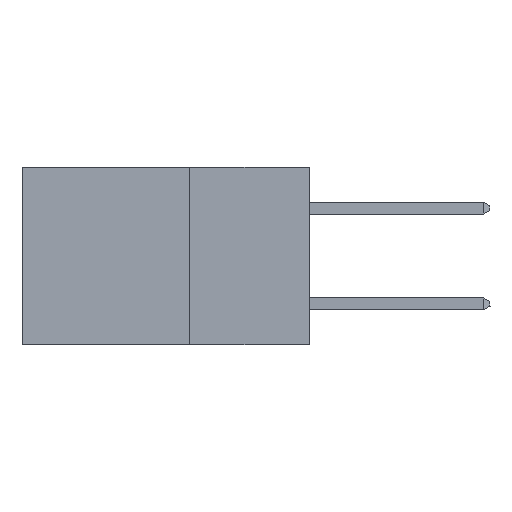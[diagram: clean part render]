
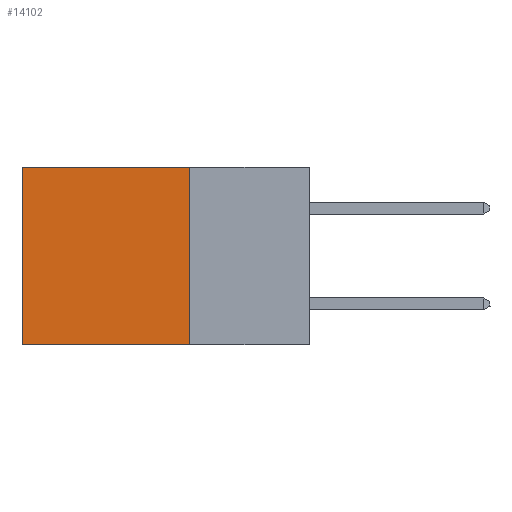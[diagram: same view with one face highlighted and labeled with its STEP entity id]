
A CAD part, left-side view. The second image highlights one B-rep face of the part: STEP entity #14102.
In plain terms, the highlighted planar face has unit normal (-1, 0, 0).
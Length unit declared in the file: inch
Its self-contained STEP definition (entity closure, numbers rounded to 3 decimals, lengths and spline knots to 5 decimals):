
#284 = VERTEX_POINT ( 'NONE', #14737 ) ;
#2550 = LINE ( 'NONE', #11551, #12801 ) ;
#3171 = ORIENTED_EDGE ( 'NONE', *, *, #9326, .T. ) ;
#3224 = ORIENTED_EDGE ( 'NONE', *, *, #5457, .F. ) ;
#3349 = ORIENTED_EDGE ( 'NONE', *, *, #16497, .F. ) ;
#3439 = CARTESIAN_POINT ( 'NONE',  ( 0.2875, 0.25, -0.37 ) ) ;
#3524 = CARTESIAN_POINT ( 'NONE',  ( 0.2875, 0.25, -0.37 ) ) ;
#4441 = AXIS2_PLACEMENT_3D ( 'NONE', #5924, #4626, #13825 ) ;
#4534 = EDGE_CURVE ( 'NONE', #12306, #284, #9632, .T. ) ;
#4618 = DIRECTION ( 'NONE',  ( 0., 1., 0. ) ) ;
#4626 = DIRECTION ( 'NONE',  ( 1., 0., 0. ) ) ;
#4985 = DIRECTION ( 'NONE',  ( 0., 0., -1. ) ) ;
#5374 = ORIENTED_EDGE ( 'NONE', *, *, #4534, .T. ) ;
#5457 = EDGE_CURVE ( 'NONE', #10464, #12548, #16522, .T. ) ;
#5924 = CARTESIAN_POINT ( 'NONE',  ( 0.2875, 0.25, 0. ) ) ;
#6293 = DIRECTION ( 'NONE',  ( 0., 0., -1. ) ) ;
#8599 = PLANE ( 'NONE',  #4441 ) ;
#9233 = VECTOR ( 'NONE', #10150, 39.37008 ) ;
#9326 = EDGE_CURVE ( 'NONE', #284, #12548, #11108, .T. ) ;
#9632 = LINE ( 'NONE', #10018, #9233 ) ;
#10004 = CARTESIAN_POINT ( 'NONE',  ( 0.2875, 0.25, 0. ) ) ;
#10018 = CARTESIAN_POINT ( 'NONE',  ( 0.2875, 0.25, 0. ) ) ;
#10150 = DIRECTION ( 'NONE',  ( 0., 1., 0. ) ) ;
#10243 = EDGE_LOOP ( 'NONE', ( #3171, #3224, #3349, #5374 ) ) ;
#10464 = VERTEX_POINT ( 'NONE', #3439 ) ;
#11108 = LINE ( 'NONE', #11482, #11503 ) ;
#11482 = CARTESIAN_POINT ( 'NONE',  ( 0.2875, 0.6, 0. ) ) ;
#11503 = VECTOR ( 'NONE', #6293, 39.37008 ) ;
#11551 = CARTESIAN_POINT ( 'NONE',  ( 0.2875, 0.25, 0. ) ) ;
#12306 = VERTEX_POINT ( 'NONE', #10004 ) ;
#12548 = VERTEX_POINT ( 'NONE', #13087 ) ;
#12668 = VECTOR ( 'NONE', #4618, 39.37008 ) ;
#12801 = VECTOR ( 'NONE', #4985, 39.37008 ) ;
#13087 = CARTESIAN_POINT ( 'NONE',  ( 0.2875, 0.6, -0.37 ) ) ;
#13478 = FACE_OUTER_BOUND ( 'NONE', #10243, .T. ) ;
#13825 = DIRECTION ( 'NONE',  ( 0., 0., -1. ) ) ;
#14102 = ADVANCED_FACE ( 'NONE', ( #13478 ), #8599, .F. ) ;
#14737 = CARTESIAN_POINT ( 'NONE',  ( 0.2875, 0.6, 0. ) ) ;
#16497 = EDGE_CURVE ( 'NONE', #12306, #10464, #2550, .T. ) ;
#16522 = LINE ( 'NONE', #3524, #12668 ) ;
